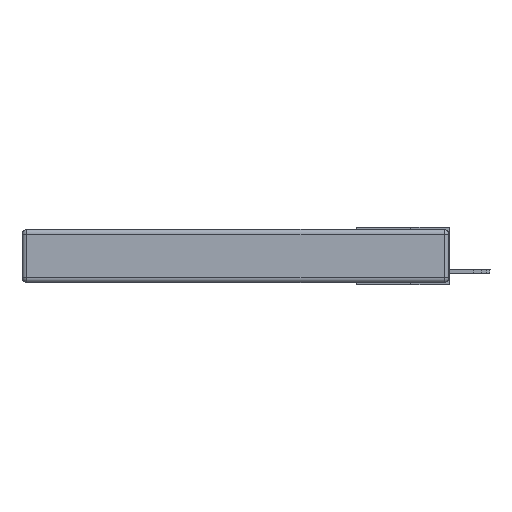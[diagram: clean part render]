
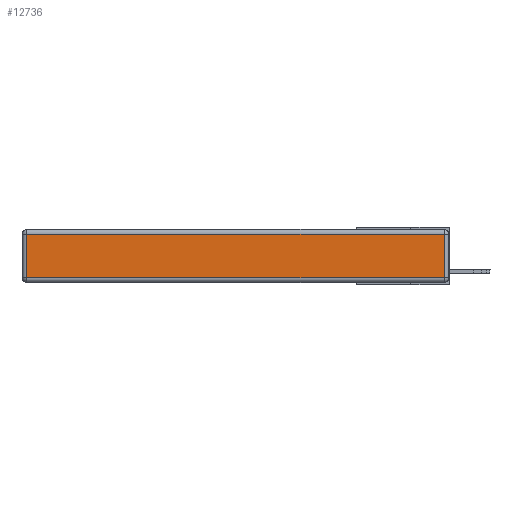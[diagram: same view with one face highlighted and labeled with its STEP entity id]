
A CAD part, left-side view. The second image highlights one B-rep face of the part: STEP entity #12736.
In plain terms, the highlighted planar face has unit normal (-1, 0, 0).
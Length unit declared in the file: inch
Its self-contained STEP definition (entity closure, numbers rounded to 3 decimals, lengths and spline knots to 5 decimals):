
#582 = EDGE_LOOP ( 'NONE', ( #17502, #6157, #19396, #10914 ) ) ;
#1305 = CARTESIAN_POINT ( 'NONE',  ( 0., 0.03, -0.313 ) ) ;
#2234 = EDGE_CURVE ( 'NONE', #10825, #12593, #7120, .T. ) ;
#2583 = DIRECTION ( 'NONE',  ( 0., 1., 0. ) ) ;
#3076 = VECTOR ( 'NONE', #14486, 39.37008 ) ;
#3686 = LINE ( 'NONE', #17794, #12081 ) ;
#3913 = CARTESIAN_POINT ( 'NONE',  ( 0., 0., -0.313 ) ) ;
#4004 = FACE_OUTER_BOUND ( 'NONE', #582, .T. ) ;
#5581 = CARTESIAN_POINT ( 'NONE',  ( 0., 0., -0.343 ) ) ;
#5846 = DIRECTION ( 'NONE',  ( 0., 0., 1. ) ) ;
#6157 = ORIENTED_EDGE ( 'NONE', *, *, #15075, .T. ) ;
#6928 = DIRECTION ( 'NONE',  ( 0., 0., -1. ) ) ;
#7120 = LINE ( 'NONE', #3913, #3076 ) ;
#8163 = EDGE_CURVE ( 'NONE', #14478, #9807, #10398, .T. ) ;
#8472 = AXIS2_PLACEMENT_3D ( 'NONE', #5581, #8749, #5846 ) ;
#8654 = DIRECTION ( 'NONE',  ( 0., 0., 1. ) ) ;
#8749 = DIRECTION ( 'NONE',  ( -1., 0., 0. ) ) ;
#9704 = VECTOR ( 'NONE', #6928, 39.37008 ) ;
#9807 = VERTEX_POINT ( 'NONE', #15414 ) ;
#10398 = LINE ( 'NONE', #19438, #17556 ) ;
#10825 = VERTEX_POINT ( 'NONE', #12348 ) ;
#10914 = ORIENTED_EDGE ( 'NONE', *, *, #13064, .T. ) ;
#12081 = VECTOR ( 'NONE', #8654, 39.37008 ) ;
#12348 = CARTESIAN_POINT ( 'NONE',  ( 0., 2.72, -0.313 ) ) ;
#12593 = VERTEX_POINT ( 'NONE', #1305 ) ;
#12736 = ADVANCED_FACE ( 'NONE', ( #4004 ), #14592, .T. ) ;
#13064 = EDGE_CURVE ( 'NONE', #9807, #10825, #16371, .T. ) ;
#14478 = VERTEX_POINT ( 'NONE', #16071 ) ;
#14486 = DIRECTION ( 'NONE',  ( 0., -1., 0. ) ) ;
#14592 = PLANE ( 'NONE',  #8472 ) ;
#15075 = EDGE_CURVE ( 'NONE', #12593, #14478, #3686, .T. ) ;
#15414 = CARTESIAN_POINT ( 'NONE',  ( 0., 2.72, -0.03 ) ) ;
#16071 = CARTESIAN_POINT ( 'NONE',  ( 0., 0.03, -0.03 ) ) ;
#16371 = LINE ( 'NONE', #19296, #9704 ) ;
#17502 = ORIENTED_EDGE ( 'NONE', *, *, #2234, .T. ) ;
#17556 = VECTOR ( 'NONE', #2583, 39.37008 ) ;
#17794 = CARTESIAN_POINT ( 'NONE',  ( 0., 0.03, -0.343 ) ) ;
#19296 = CARTESIAN_POINT ( 'NONE',  ( 0., 2.72, -0.343 ) ) ;
#19396 = ORIENTED_EDGE ( 'NONE', *, *, #8163, .T. ) ;
#19438 = CARTESIAN_POINT ( 'NONE',  ( 0., 2.75, -0.03 ) ) ;
